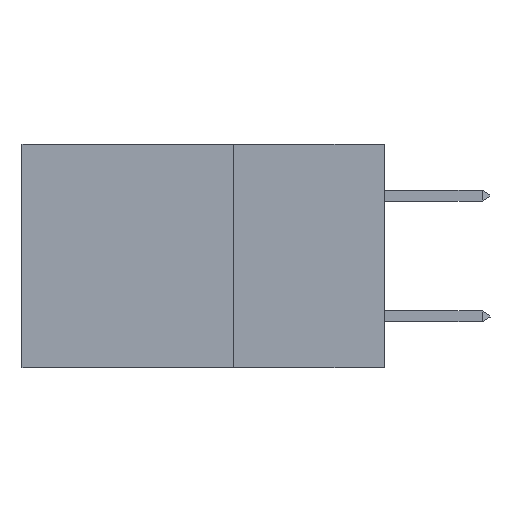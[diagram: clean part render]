
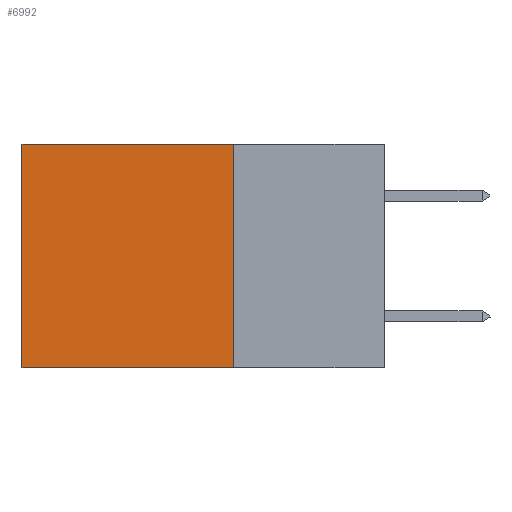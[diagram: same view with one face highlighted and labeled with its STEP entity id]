
A CAD part, left-side view. The second image highlights one B-rep face of the part: STEP entity #6992.
In plain terms, the highlighted planar face has unit normal (-1, 0, 0).
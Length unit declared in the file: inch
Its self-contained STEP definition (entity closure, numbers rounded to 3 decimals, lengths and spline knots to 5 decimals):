
#539 = VECTOR ( 'NONE', #8020, 39.37008 ) ;
#649 = CARTESIAN_POINT ( 'NONE',  ( 0.2875, 0.25, 0. ) ) ;
#981 = VERTEX_POINT ( 'NONE', #10938 ) ;
#1441 = DIRECTION ( 'NONE',  ( 0., 1., 0. ) ) ;
#1551 = LINE ( 'NONE', #5883, #14103 ) ;
#2099 = ORIENTED_EDGE ( 'NONE', *, *, #3113, .F. ) ;
#2144 = CARTESIAN_POINT ( 'NONE',  ( 0.2875, 0.25, 0. ) ) ;
#2271 = DIRECTION ( 'NONE',  ( 0., 0., -1. ) ) ;
#2933 = ORIENTED_EDGE ( 'NONE', *, *, #6208, .F. ) ;
#3113 = EDGE_CURVE ( 'NONE', #11418, #7255, #1551, .T. ) ;
#3197 = CARTESIAN_POINT ( 'NONE',  ( 0.2875, 0.25, -0.37 ) ) ;
#3286 = CARTESIAN_POINT ( 'NONE',  ( 0.2875, 0.25, 0. ) ) ;
#3568 = CARTESIAN_POINT ( 'NONE',  ( 0.2875, 0.6, -0.37 ) ) ;
#4872 = EDGE_LOOP ( 'NONE', ( #8624, #2099, #2933, #8131 ) ) ;
#5362 = DIRECTION ( 'NONE',  ( 0., 0., -1. ) ) ;
#5421 = FACE_OUTER_BOUND ( 'NONE', #4872, .T. ) ;
#5883 = CARTESIAN_POINT ( 'NONE',  ( 0.2875, 0.25, -0.37 ) ) ;
#6104 = VECTOR ( 'NONE', #2271, 39.37008 ) ;
#6208 = EDGE_CURVE ( 'NONE', #13189, #11418, #12314, .T. ) ;
#6222 = DIRECTION ( 'NONE',  ( 1., 0., 0. ) ) ;
#6992 = ADVANCED_FACE ( 'NONE', ( #5421 ), #11775, .F. ) ;
#7255 = VERTEX_POINT ( 'NONE', #3568 ) ;
#7898 = CARTESIAN_POINT ( 'NONE',  ( 0.2875, 0.25, 0. ) ) ;
#8020 = DIRECTION ( 'NONE',  ( 0., 1., 0. ) ) ;
#8131 = ORIENTED_EDGE ( 'NONE', *, *, #9439, .T. ) ;
#8592 = CARTESIAN_POINT ( 'NONE',  ( 0.2875, 0.6, 0. ) ) ;
#8624 = ORIENTED_EDGE ( 'NONE', *, *, #13452, .T. ) ;
#9439 = EDGE_CURVE ( 'NONE', #13189, #981, #9984, .T. ) ;
#9984 = LINE ( 'NONE', #7898, #539 ) ;
#10938 = CARTESIAN_POINT ( 'NONE',  ( 0.2875, 0.6, 0. ) ) ;
#10961 = AXIS2_PLACEMENT_3D ( 'NONE', #2144, #6222, #11967 ) ;
#11027 = VECTOR ( 'NONE', #5362, 39.37008 ) ;
#11418 = VERTEX_POINT ( 'NONE', #3197 ) ;
#11775 = PLANE ( 'NONE',  #10961 ) ;
#11967 = DIRECTION ( 'NONE',  ( 0., 0., -1. ) ) ;
#12072 = LINE ( 'NONE', #8592, #11027 ) ;
#12314 = LINE ( 'NONE', #3286, #6104 ) ;
#13189 = VERTEX_POINT ( 'NONE', #649 ) ;
#13452 = EDGE_CURVE ( 'NONE', #981, #7255, #12072, .T. ) ;
#14103 = VECTOR ( 'NONE', #1441, 39.37008 ) ;
